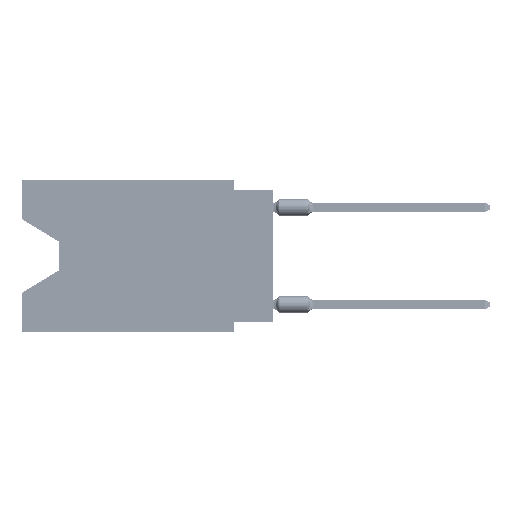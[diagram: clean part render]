
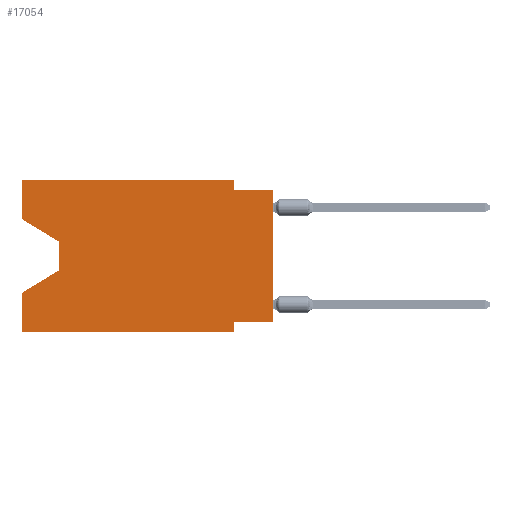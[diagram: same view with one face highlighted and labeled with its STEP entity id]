
A CAD part, left-side view. The second image highlights one B-rep face of the part: STEP entity #17054.
In plain terms, the highlighted planar face has unit normal (-1, 0, 0).
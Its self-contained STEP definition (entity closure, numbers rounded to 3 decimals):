
#553 = LINE ( 'NONE', #51347, #55809 ) ;
#564 = VECTOR ( 'NONE', #66677, 1000. ) ;
#883 = VERTEX_POINT ( 'NONE', #3503 ) ;
#1380 = LINE ( 'NONE', #40686, #43027 ) ;
#2017 = DIRECTION ( 'NONE',  ( 0., -0.855, -0.519 ) ) ;
#2524 = CARTESIAN_POINT ( 'NONE',  ( 0., 0., 0. ) ) ;
#3503 = CARTESIAN_POINT ( 'NONE',  ( 0., 0., -0.635 ) ) ;
#3724 = DIRECTION ( 'NONE',  ( 0., 1., 0. ) ) ;
#4064 = VECTOR ( 'NONE', #35991, 1000. ) ;
#4253 = VERTEX_POINT ( 'NONE', #58001 ) ;
#4871 = CARTESIAN_POINT ( 'NONE',  ( 0., 16.383, 0. ) ) ;
#5028 = CARTESIAN_POINT ( 'NONE',  ( 0., 2.54, -0.635 ) ) ;
#5732 = VERTEX_POINT ( 'NONE', #68679 ) ;
#5829 = CARTESIAN_POINT ( 'NONE',  ( 0., 13.97, -4.013 ) ) ;
#7195 = ORIENTED_EDGE ( 'NONE', *, *, #10811, .F. ) ;
#7665 = AXIS2_PLACEMENT_3D ( 'NONE', #67920, #40512, #68659 ) ;
#8992 = CARTESIAN_POINT ( 'NONE',  ( 0., 13.97, -4.013 ) ) ;
#10025 = CARTESIAN_POINT ( 'NONE',  ( 0., 2.54, -9.271 ) ) ;
#10426 = VERTEX_POINT ( 'NONE', #18194 ) ;
#10811 = EDGE_CURVE ( 'NONE', #71975, #10426, #71853, .T. ) ;
#11643 = VECTOR ( 'NONE', #16220, 1000. ) ;
#12236 = CARTESIAN_POINT ( 'NONE',  ( 0., 13.97, -5.893 ) ) ;
#14200 = VERTEX_POINT ( 'NONE', #4871 ) ;
#16220 = DIRECTION ( 'NONE',  ( 0., -1., 0. ) ) ;
#17054 = ADVANCED_FACE ( 'NONE', ( #44600 ), #67561, .F. ) ;
#18194 = CARTESIAN_POINT ( 'NONE',  ( 0., 2.54, -9.906 ) ) ;
#18222 = LINE ( 'NONE', #47474, #4064 ) ;
#19142 = CARTESIAN_POINT ( 'NONE',  ( 0., 13.97, -5.893 ) ) ;
#19989 = VECTOR ( 'NONE', #41748, 1000. ) ;
#20009 = VERTEX_POINT ( 'NONE', #31946 ) ;
#20734 = VECTOR ( 'NONE', #41109, 1000. ) ;
#22097 = EDGE_CURVE ( 'NONE', #35272, #14200, #24197, .T. ) ;
#23107 = CARTESIAN_POINT ( 'NONE',  ( 0., 16.383, 0. ) ) ;
#23181 = DIRECTION ( 'NONE',  ( 0., -1., 0. ) ) ;
#24197 = LINE ( 'NONE', #23107, #60171 ) ;
#25893 = ORIENTED_EDGE ( 'NONE', *, *, #55293, .T. ) ;
#26669 = VECTOR ( 'NONE', #3724, 1000. ) ;
#30211 = LINE ( 'NONE', #52799, #68558 ) ;
#30351 = VERTEX_POINT ( 'NONE', #12236 ) ;
#30368 = LINE ( 'NONE', #57778, #20734 ) ;
#31666 = DIRECTION ( 'NONE',  ( 0., 0., -1. ) ) ;
#31946 = CARTESIAN_POINT ( 'NONE',  ( 0., 2.54, 0. ) ) ;
#32001 = VERTEX_POINT ( 'NONE', #65804 ) ;
#32864 = DIRECTION ( 'NONE',  ( 0., 0., 1. ) ) ;
#33644 = CARTESIAN_POINT ( 'NONE',  ( 0., 16.383, -9.906 ) ) ;
#34739 = EDGE_CURVE ( 'NONE', #20009, #73055, #1380, .T. ) ;
#35272 = VERTEX_POINT ( 'NONE', #71195 ) ;
#35991 = DIRECTION ( 'NONE',  ( 0., 0., 1. ) ) ;
#36187 = LINE ( 'NONE', #19142, #19989 ) ;
#36326 = ORIENTED_EDGE ( 'NONE', *, *, #43180, .T. ) ;
#36347 = ORIENTED_EDGE ( 'NONE', *, *, #60876, .F. ) ;
#40512 = DIRECTION ( 'NONE',  ( 1., 0., 0. ) ) ;
#40686 = CARTESIAN_POINT ( 'NONE',  ( 0., 2.54, 0. ) ) ;
#41109 = DIRECTION ( 'NONE',  ( 0., -1., 0. ) ) ;
#41748 = DIRECTION ( 'NONE',  ( 0., 0.855, -0.519 ) ) ;
#42668 = CARTESIAN_POINT ( 'NONE',  ( 0., 0., -9.271 ) ) ;
#43027 = VECTOR ( 'NONE', #31666, 1000. ) ;
#43180 = EDGE_CURVE ( 'NONE', #35272, #57964, #30211, .T. ) ;
#43457 = ORIENTED_EDGE ( 'NONE', *, *, #71905, .F. ) ;
#44600 = FACE_OUTER_BOUND ( 'NONE', #64203, .T. ) ;
#45750 = ORIENTED_EDGE ( 'NONE', *, *, #52087, .T. ) ;
#45934 = ORIENTED_EDGE ( 'NONE', *, *, #34739, .F. ) ;
#47474 = CARTESIAN_POINT ( 'NONE',  ( 0., 16.383, 0. ) ) ;
#47746 = DIRECTION ( 'NONE',  ( 0., 0., 1. ) ) ;
#50927 = ORIENTED_EDGE ( 'NONE', *, *, #72257, .F. ) ;
#51186 = ORIENTED_EDGE ( 'NONE', *, *, #52531, .T. ) ;
#51347 = CARTESIAN_POINT ( 'NONE',  ( 0., 16.383, 0. ) ) ;
#52087 = EDGE_CURVE ( 'NONE', #4253, #883, #53314, .T. ) ;
#52245 = EDGE_CURVE ( 'NONE', #5732, #10426, #71792, .T. ) ;
#52531 = EDGE_CURVE ( 'NONE', #30351, #32001, #36187, .T. ) ;
#52735 = ORIENTED_EDGE ( 'NONE', *, *, #70569, .F. ) ;
#52799 = CARTESIAN_POINT ( 'NONE',  ( 0., 16.383, -2.546 ) ) ;
#53314 = LINE ( 'NONE', #2524, #66066 ) ;
#54453 = ORIENTED_EDGE ( 'NONE', *, *, #52245, .T. ) ;
#54871 = LINE ( 'NONE', #42668, #26669 ) ;
#55293 = EDGE_CURVE ( 'NONE', #57964, #30351, #70873, .T. ) ;
#55809 = VECTOR ( 'NONE', #23181, 1000. ) ;
#57580 = ORIENTED_EDGE ( 'NONE', *, *, #22097, .F. ) ;
#57778 = CARTESIAN_POINT ( 'NONE',  ( 0., 0., -0.635 ) ) ;
#57964 = VERTEX_POINT ( 'NONE', #5829 ) ;
#58001 = CARTESIAN_POINT ( 'NONE',  ( 0., 0., -9.271 ) ) ;
#60171 = VECTOR ( 'NONE', #32864, 1000. ) ;
#60501 = DIRECTION ( 'NONE',  ( 0., 0., -1. ) ) ;
#60876 = EDGE_CURVE ( 'NONE', #14200, #20009, #553, .T. ) ;
#64203 = EDGE_LOOP ( 'NONE', ( #36326, #25893, #51186, #52735, #54453, #7195, #43457, #45750, #50927, #45934, #36347, #57580 ) ) ;
#65804 = CARTESIAN_POINT ( 'NONE',  ( 0., 16.383, -7.36 ) ) ;
#66066 = VECTOR ( 'NONE', #47746, 1000. ) ;
#66319 = CARTESIAN_POINT ( 'NONE',  ( 0., 2.54, -9.906 ) ) ;
#66677 = DIRECTION ( 'NONE',  ( 0., 0., -1. ) ) ;
#67561 = PLANE ( 'NONE',  #7665 ) ;
#67920 = CARTESIAN_POINT ( 'NONE',  ( 0., 16.383, 0. ) ) ;
#68558 = VECTOR ( 'NONE', #2017, 1000. ) ;
#68659 = DIRECTION ( 'NONE',  ( 0., 0., -1. ) ) ;
#68679 = CARTESIAN_POINT ( 'NONE',  ( 0., 16.383, -9.906 ) ) ;
#69450 = VECTOR ( 'NONE', #60501, 1000. ) ;
#70569 = EDGE_CURVE ( 'NONE', #5732, #32001, #18222, .T. ) ;
#70873 = LINE ( 'NONE', #8992, #69450 ) ;
#71195 = CARTESIAN_POINT ( 'NONE',  ( 0., 16.383, -2.546 ) ) ;
#71792 = LINE ( 'NONE', #33644, #11643 ) ;
#71853 = LINE ( 'NONE', #66319, #564 ) ;
#71905 = EDGE_CURVE ( 'NONE', #4253, #71975, #54871, .T. ) ;
#71975 = VERTEX_POINT ( 'NONE', #10025 ) ;
#72257 = EDGE_CURVE ( 'NONE', #73055, #883, #30368, .T. ) ;
#73055 = VERTEX_POINT ( 'NONE', #5028 ) ;
